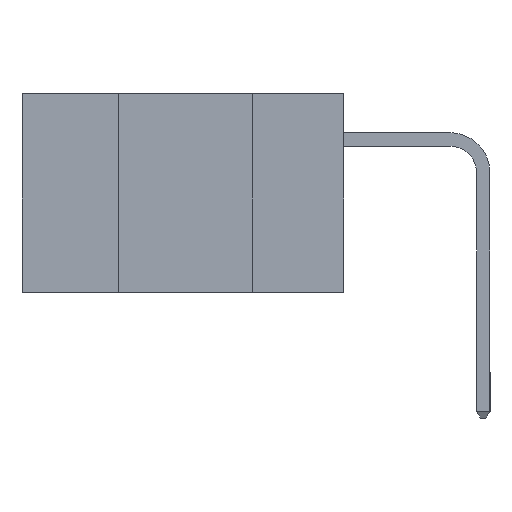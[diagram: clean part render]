
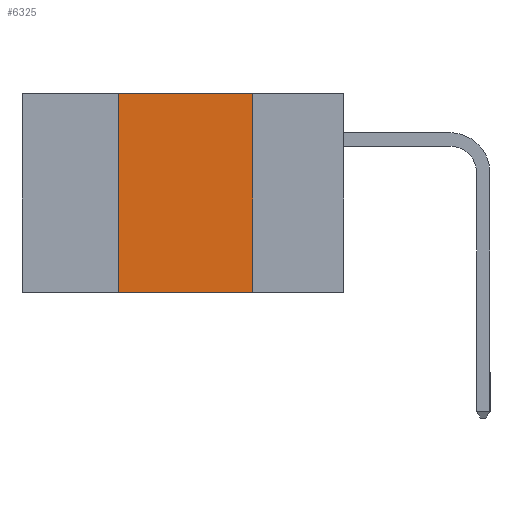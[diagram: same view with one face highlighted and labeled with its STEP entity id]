
A CAD part, left-side view. The second image highlights one B-rep face of the part: STEP entity #6325.
In plain terms, the highlighted planar face has unit normal (-1, 0, 0).
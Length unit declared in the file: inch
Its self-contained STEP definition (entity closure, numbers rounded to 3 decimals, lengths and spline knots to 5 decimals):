
#179 = ORIENTED_EDGE ( 'NONE', *, *, #9291, .F. ) ;
#285 = LINE ( 'NONE', #9051, #3571 ) ;
#294 = VECTOR ( 'NONE', #5118, 39.37008 ) ;
#609 = DIRECTION ( 'NONE',  ( 0., 0., 1. ) ) ;
#900 = VERTEX_POINT ( 'NONE', #6532 ) ;
#1478 = EDGE_CURVE ( 'NONE', #3961, #900, #8794, .T. ) ;
#1644 = CARTESIAN_POINT ( 'NONE',  ( 0., 0.6, -0.37 ) ) ;
#1972 = VERTEX_POINT ( 'NONE', #7408 ) ;
#2194 = CARTESIAN_POINT ( 'NONE',  ( 0., 0.17, -0.37 ) ) ;
#2392 = VERTEX_POINT ( 'NONE', #2569 ) ;
#2569 = CARTESIAN_POINT ( 'NONE',  ( 0., 0.42, 0. ) ) ;
#2905 = CARTESIAN_POINT ( 'NONE',  ( 0., 0.17, 0. ) ) ;
#3091 = LINE ( 'NONE', #1644, #6952 ) ;
#3157 = DIRECTION ( 'NONE',  ( 0., 0., -1. ) ) ;
#3433 = VECTOR ( 'NONE', #609, 39.37008 ) ;
#3559 = CARTESIAN_POINT ( 'NONE',  ( 0., 0.42, -0.37 ) ) ;
#3571 = VECTOR ( 'NONE', #7556, 39.37008 ) ;
#3961 = VERTEX_POINT ( 'NONE', #2905 ) ;
#4276 = LINE ( 'NONE', #3559, #3433 ) ;
#4517 = ORIENTED_EDGE ( 'NONE', *, *, #7960, .F. ) ;
#4595 = FACE_OUTER_BOUND ( 'NONE', #6062, .T. ) ;
#4608 = AXIS2_PLACEMENT_3D ( 'NONE', #5272, #8852, #3157 ) ;
#5118 = DIRECTION ( 'NONE',  ( 0., 0., -1. ) ) ;
#5272 = CARTESIAN_POINT ( 'NONE',  ( 0., 0.6, 0. ) ) ;
#5930 = DIRECTION ( 'NONE',  ( 0., -1., 0. ) ) ;
#6062 = EDGE_LOOP ( 'NONE', ( #7317, #4517, #179, #7124 ) ) ;
#6325 = ADVANCED_FACE ( 'NONE', ( #4595 ), #7542, .F. ) ;
#6532 = CARTESIAN_POINT ( 'NONE',  ( 0., 0.17, -0.37 ) ) ;
#6952 = VECTOR ( 'NONE', #5930, 39.37008 ) ;
#7124 = ORIENTED_EDGE ( 'NONE', *, *, #8645, .T. ) ;
#7317 = ORIENTED_EDGE ( 'NONE', *, *, #1478, .F. ) ;
#7408 = CARTESIAN_POINT ( 'NONE',  ( 0., 0.42, -0.37 ) ) ;
#7542 = PLANE ( 'NONE',  #4608 ) ;
#7556 = DIRECTION ( 'NONE',  ( 0., -1., 0. ) ) ;
#7960 = EDGE_CURVE ( 'NONE', #2392, #3961, #285, .T. ) ;
#8645 = EDGE_CURVE ( 'NONE', #1972, #900, #3091, .T. ) ;
#8794 = LINE ( 'NONE', #2194, #294 ) ;
#8852 = DIRECTION ( 'NONE',  ( 1., 0., 0. ) ) ;
#9051 = CARTESIAN_POINT ( 'NONE',  ( 0., 0.6, 0. ) ) ;
#9291 = EDGE_CURVE ( 'NONE', #1972, #2392, #4276, .T. ) ;
